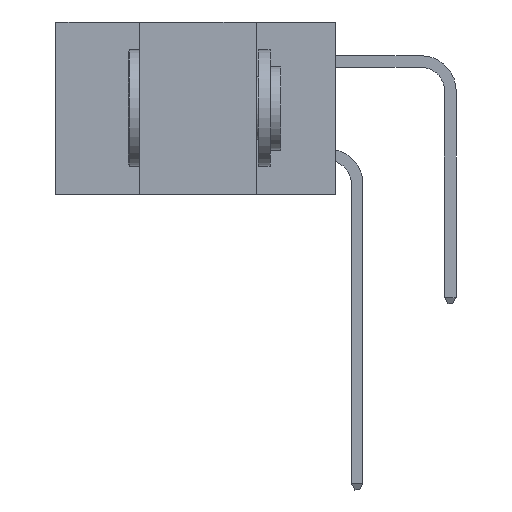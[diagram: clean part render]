
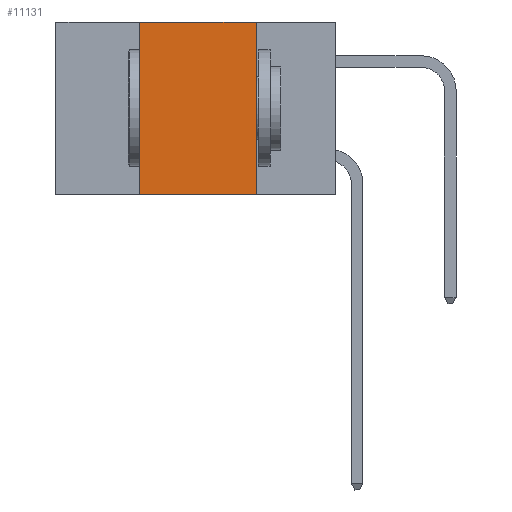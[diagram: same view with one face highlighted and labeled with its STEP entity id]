
A CAD part, left-side view. The second image highlights one B-rep face of the part: STEP entity #11131.
In plain terms, the highlighted planar face has unit normal (-1, 0, 0).
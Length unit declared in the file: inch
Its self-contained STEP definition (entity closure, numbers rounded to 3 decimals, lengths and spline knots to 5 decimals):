
#682 = AXIS2_PLACEMENT_3D ( 'NONE', #19460, #1693, #9429 ) ;
#840 = CARTESIAN_POINT ( 'NONE',  ( 0., 0.17, -0.37 ) ) ;
#1120 = DIRECTION ( 'NONE',  ( 0., -1., 0. ) ) ;
#1693 = DIRECTION ( 'NONE',  ( 1., 0., 0. ) ) ;
#2637 = ORIENTED_EDGE ( 'NONE', *, *, #20926, .F. ) ;
#3568 = VECTOR ( 'NONE', #5708, 39.37008 ) ;
#4778 = VERTEX_POINT ( 'NONE', #8914 ) ;
#5708 = DIRECTION ( 'NONE',  ( 0., -1., 0. ) ) ;
#5983 = PLANE ( 'NONE',  #682 ) ;
#7115 = LINE ( 'NONE', #25250, #3568 ) ;
#7642 = CARTESIAN_POINT ( 'NONE',  ( 0., 0.17, 0. ) ) ;
#8281 = VERTEX_POINT ( 'NONE', #26454 ) ;
#8869 = LINE ( 'NONE', #20946, #25921 ) ;
#8914 = CARTESIAN_POINT ( 'NONE',  ( 0., 0.42, 0. ) ) ;
#8993 = VERTEX_POINT ( 'NONE', #12433 ) ;
#9164 = EDGE_CURVE ( 'NONE', #4778, #8281, #8869, .T. ) ;
#9429 = DIRECTION ( 'NONE',  ( 0., 0., -1. ) ) ;
#9446 = ORIENTED_EDGE ( 'NONE', *, *, #9164, .F. ) ;
#9694 = EDGE_CURVE ( 'NONE', #8993, #4778, #18296, .T. ) ;
#11131 = ADVANCED_FACE ( 'NONE', ( #12613 ), #5983, .F. ) ;
#11541 = ORIENTED_EDGE ( 'NONE', *, *, #9694, .F. ) ;
#12268 = VERTEX_POINT ( 'NONE', #840 ) ;
#12433 = CARTESIAN_POINT ( 'NONE',  ( 0., 0.42, -0.37 ) ) ;
#12613 = FACE_OUTER_BOUND ( 'NONE', #18944, .T. ) ;
#15788 = VECTOR ( 'NONE', #27877, 39.37008 ) ;
#17876 = LINE ( 'NONE', #7642, #15788 ) ;
#18296 = LINE ( 'NONE', #20446, #22098 ) ;
#18944 = EDGE_LOOP ( 'NONE', ( #2637, #9446, #11541, #21080 ) ) ;
#19460 = CARTESIAN_POINT ( 'NONE',  ( 0., 0.6, 0. ) ) ;
#20446 = CARTESIAN_POINT ( 'NONE',  ( 0., 0.42, 0. ) ) ;
#20926 = EDGE_CURVE ( 'NONE', #8281, #12268, #17876, .T. ) ;
#20946 = CARTESIAN_POINT ( 'NONE',  ( 0., 0.6, 0. ) ) ;
#21080 = ORIENTED_EDGE ( 'NONE', *, *, #25224, .T. ) ;
#22098 = VECTOR ( 'NONE', #22874, 39.37008 ) ;
#22874 = DIRECTION ( 'NONE',  ( 0., 0., 1. ) ) ;
#25224 = EDGE_CURVE ( 'NONE', #8993, #12268, #7115, .T. ) ;
#25250 = CARTESIAN_POINT ( 'NONE',  ( 0., 0.6, -0.37 ) ) ;
#25921 = VECTOR ( 'NONE', #1120, 39.37008 ) ;
#26454 = CARTESIAN_POINT ( 'NONE',  ( 0., 0.17, 0. ) ) ;
#27877 = DIRECTION ( 'NONE',  ( 0., 0., -1. ) ) ;
